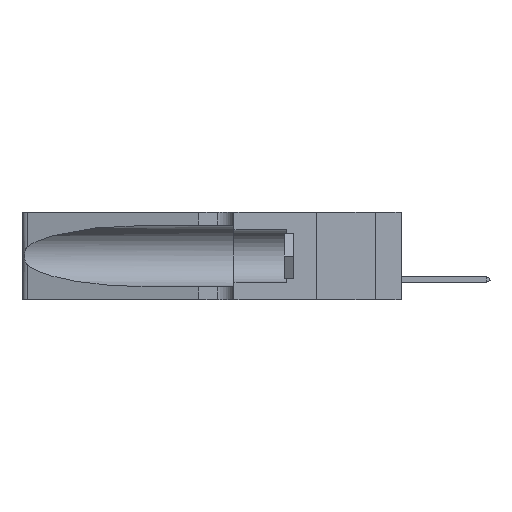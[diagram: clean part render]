
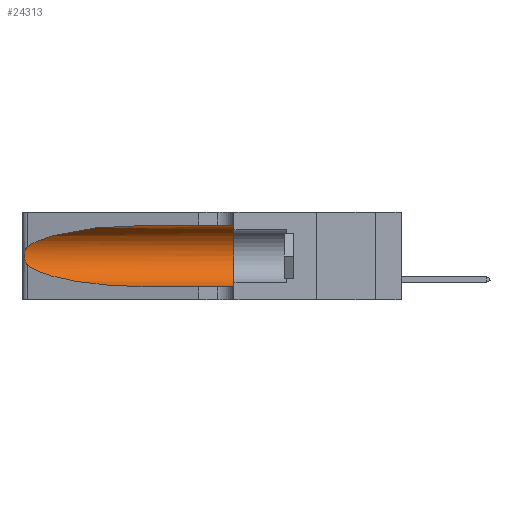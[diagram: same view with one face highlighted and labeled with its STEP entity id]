
A CAD part, left-side view. The second image highlights one B-rep face of the part: STEP entity #24313.
In plain terms, the highlighted cylindrical face has radius 3.308 mm (diameter 6.617 mm), a partial arc.
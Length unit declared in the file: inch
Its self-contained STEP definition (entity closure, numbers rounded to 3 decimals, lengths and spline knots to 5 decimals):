
#214 = DIRECTION ( 'NONE',  ( 0., 0., 1. ) ) ;
#429 = CARTESIAN_POINT ( 'NONE',  ( 0.25854, 1.2359, 0.20912 ) ) ;
#515 = CARTESIAN_POINT ( 'NONE',  ( 0.25487, 1.22718, 0.14631 ) ) ;
#635 = CARTESIAN_POINT ( 'NONE',  ( 0.25487, 1.22718, 0.22369 ) ) ;
#1955 = LINE ( 'NONE', #13099, #14165 ) ;
#2185 = CYLINDRICAL_SURFACE ( 'NONE', #22922, 0.13025 ) ;
#2389 = CARTESIAN_POINT ( 'NONE',  ( 0.25856, 1.23593, 0.16098 ) ) ;
#2677 = CARTESIAN_POINT ( 'NONE',  ( 0.1305, 0.72297, 0.31525 ) ) ;
#3115 = DIRECTION ( 'NONE',  ( 0., -1., 0. ) ) ;
#3219 = VERTEX_POINT ( 'NONE', #7166 ) ;
#3462 = EDGE_CURVE ( 'NONE', #11385, #7246, #1955, .T. ) ;
#4163 = CARTESIAN_POINT ( 'NONE',  ( 0.25555, 1.22994, 0.2215 ) ) ;
#4325 = CARTESIAN_POINT ( 'NONE',  ( 0.25555, 1.22993, 0.14849 ) ) ;
#4546 = CARTESIAN_POINT ( 'NONE',  ( 0.1305, 0.35, 0.31525 ) ) ;
#4850 = EDGE_CURVE ( 'NONE', #7246, #5828, #12979, .T. ) ;
#5003 = VERTEX_POINT ( 'NONE', #515 ) ;
#5812 = EDGE_CURVE ( 'NONE', #24783, #5003, #18375, .T. ) ;
#5828 = VERTEX_POINT ( 'NONE', #21997 ) ;
#6577 = CARTESIAN_POINT ( 'NONE',  ( 0.2373, 1.15595, 0.28018 ) ) ;
#6767 = CARTESIAN_POINT ( 'NONE',  ( 0.18966, 0.96281, 0.05475 ) ) ;
#7166 = CARTESIAN_POINT ( 'NONE',  ( 0.1305, 0.72297, 0.05475 ) ) ;
#7246 = VERTEX_POINT ( 'NONE', #4546 ) ;
#7293 = CARTESIAN_POINT ( 'NONE',  ( 0.1305, 0.72297, 0.31525 ) ) ;
#7472 = ORIENTED_EDGE ( 'NONE', *, *, #23470, .T. ) ;
#7859 = CARTESIAN_POINT ( 'NONE',  ( 0.25487, 1.22718, 0.14631 ) ) ;
#9243 = DIRECTION ( 'NONE',  ( 0., -1., 0. ) ) ;
#9976 = CARTESIAN_POINT ( 'NONE',  ( 0.25639, 1.23184, 0.21858 ) ) ;
#10081 = DIRECTION ( 'NONE',  ( 0., -1., 0. ) ) ;
#10697 = CARTESIAN_POINT ( 'NONE',  ( 0.1305, 1.61858, 0.05475 ) ) ;
#11385 = VERTEX_POINT ( 'NONE', #7293 ) ;
#11780 = CARTESIAN_POINT ( 'NONE',  ( 0.25487, 1.22718, 0.22369 ) ) ;
#11904 = DIRECTION ( 'NONE',  ( 0., 1., 0. ) ) ;
#12109 = CARTESIAN_POINT ( 'NONE',  ( 0.26075, 1.23896, 0.178 ) ) ;
#12230 = DIRECTION ( 'NONE',  ( 0., 0., -1. ) ) ;
#12271 = FACE_OUTER_BOUND ( 'NONE', #13973, .T. ) ;
#12979 = CIRCLE ( 'NONE', #21354, 0.13025 ) ;
#13099 = CARTESIAN_POINT ( 'NONE',  ( 0.1305, 1.61858, 0.31525 ) ) ;
#13973 = EDGE_LOOP ( 'NONE', ( #15611, #19255, #7472, #17870, #18415, #20222 ) ) ;
#14098 = CARTESIAN_POINT ( 'NONE',  ( 0.26017, 1.23833, 0.17102 ) ) ;
#14155 =( BOUNDED_CURVE ( )  B_SPLINE_CURVE ( 3, ( #2677, #18476, #6577, #635 ),
 .UNSPECIFIED., .F., .F. ) 
 B_SPLINE_CURVE_WITH_KNOTS ( ( 4, 4 ),
 ( 1.5708, 2.84003 ),
 .UNSPECIFIED. ) 
 CURVE ( )  GEOMETRIC_REPRESENTATION_ITEM ( )  RATIONAL_B_SPLINE_CURVE ( ( 1., 0.87, 0.87, 1. ) ) 
 REPRESENTATION_ITEM ( '' )  );
#14165 = VECTOR ( 'NONE', #9243, 39.37008 ) ;
#14570 = CARTESIAN_POINT ( 'NONE',  ( 0.2373, 1.15595, 0.08982 ) ) ;
#15611 = ORIENTED_EDGE ( 'NONE', *, *, #18378, .T. ) ;
#15915 = CARTESIAN_POINT ( 'NONE',  ( 0.26075, 1.23896, 0.19203 ) ) ;
#16003 = CARTESIAN_POINT ( 'NONE',  ( 0.26018, 1.23835, 0.19895 ) ) ;
#16081 = CARTESIAN_POINT ( 'NONE',  ( 0.25639, 1.23186, 0.15144 ) ) ;
#16661 = VECTOR ( 'NONE', #3115, 39.37008 ) ;
#16894 = CARTESIAN_POINT ( 'NONE',  ( 0.25487, 1.22718, 0.22369 ) ) ;
#17870 = ORIENTED_EDGE ( 'NONE', *, *, #21645, .T. ) ;
#18375 = B_SPLINE_CURVE_WITH_KNOTS ( 'NONE', 3,
 ( #11780, #4163, #9976, #23654, #429, #16003, #15915, #12109, #14098, #2389, #19556, #16081, #4325, #7859 ),
 .UNSPECIFIED., .F., .F.,
 ( 4, 2, 2, 2, 2, 2, 4 ),
 ( 0., 0.00027, 0.00053, 0.00107, 0.0016, 0.00187, 0.00214 ),
 .UNSPECIFIED. ) ;
#18378 = EDGE_CURVE ( 'NONE', #11385, #24783, #14155, .T. ) ;
#18415 = ORIENTED_EDGE ( 'NONE', *, *, #4850, .F. ) ;
#18476 = CARTESIAN_POINT ( 'NONE',  ( 0.18966, 0.96281, 0.31525 ) ) ;
#19255 = ORIENTED_EDGE ( 'NONE', *, *, #5812, .T. ) ;
#19556 = CARTESIAN_POINT ( 'NONE',  ( 0.25789, 1.23486, 0.15765 ) ) ;
#20222 = ORIENTED_EDGE ( 'NONE', *, *, #3462, .F. ) ;
#20908 = LINE ( 'NONE', #10697, #16661 ) ;
#21354 = AXIS2_PLACEMENT_3D ( 'NONE', #23608, #11904, #214 ) ;
#21645 = EDGE_CURVE ( 'NONE', #3219, #5828, #20908, .T. ) ;
#21997 = CARTESIAN_POINT ( 'NONE',  ( 0.1305, 0.35, 0.05475 ) ) ;
#22922 = AXIS2_PLACEMENT_3D ( 'NONE', #23842, #10081, #12230 ) ;
#23470 = EDGE_CURVE ( 'NONE', #5003, #3219, #25128, .T. ) ;
#23608 = CARTESIAN_POINT ( 'NONE',  ( 0.1305, 0.35, 0.185 ) ) ;
#23654 = CARTESIAN_POINT ( 'NONE',  ( 0.25787, 1.23484, 0.2124 ) ) ;
#23842 = CARTESIAN_POINT ( 'NONE',  ( 0.1305, 1.61858, 0.185 ) ) ;
#24313 = ADVANCED_FACE ( 'NONE', ( #12271 ), #2185, .F. ) ;
#24464 = CARTESIAN_POINT ( 'NONE',  ( 0.25487, 1.22718, 0.14631 ) ) ;
#24648 = CARTESIAN_POINT ( 'NONE',  ( 0.1305, 0.72297, 0.05475 ) ) ;
#24783 = VERTEX_POINT ( 'NONE', #16894 ) ;
#25128 =( BOUNDED_CURVE ( )  B_SPLINE_CURVE ( 3, ( #24464, #14570, #6767, #24648 ),
 .UNSPECIFIED., .F., .T. ) 
 B_SPLINE_CURVE_WITH_KNOTS ( ( 4, 4 ),
 ( 3.44316, 4.71239 ),
 .UNSPECIFIED. ) 
 CURVE ( )  GEOMETRIC_REPRESENTATION_ITEM ( )  RATIONAL_B_SPLINE_CURVE ( ( 1., 0.87, 0.87, 1. ) ) 
 REPRESENTATION_ITEM ( '' )  );
